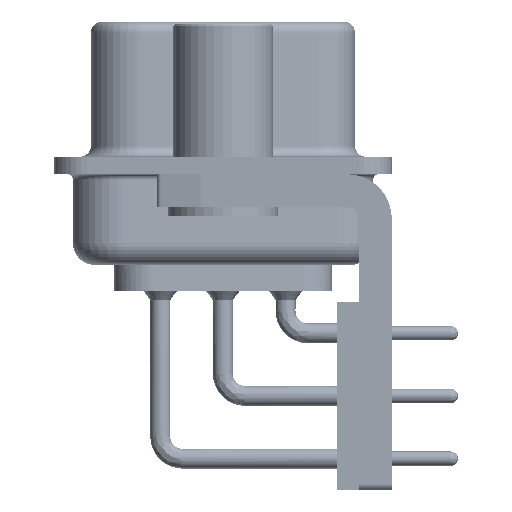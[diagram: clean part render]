
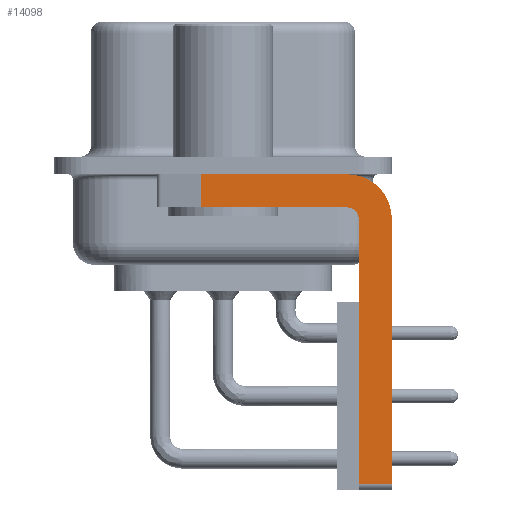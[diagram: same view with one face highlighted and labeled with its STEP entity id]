
A CAD part, left-side view. The second image highlights one B-rep face of the part: STEP entity #14098.
In plain terms, the highlighted planar face has unit normal (-1, 0, 0).
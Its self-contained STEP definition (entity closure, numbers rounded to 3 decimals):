
#279 = ORIENTED_EDGE ( 'NONE', *, *, #39820, .F. ) ;
#511 = EDGE_CURVE ( 'NONE', #20341, #10625, #32950, .T. ) ;
#591 = DIRECTION ( 'NONE',  ( -1., 0., 0. ) ) ;
#1007 = DIRECTION ( 'NONE',  ( 0., 0., -1. ) ) ;
#1360 = VERTEX_POINT ( 'NONE', #37572 ) ;
#3032 = VERTEX_POINT ( 'NONE', #11456 ) ;
#4516 = DIRECTION ( 'NONE',  ( 0., -1., 0. ) ) ;
#6173 = ORIENTED_EDGE ( 'NONE', *, *, #35330, .F. ) ;
#7024 = VECTOR ( 'NONE', #4516, 1000. ) ;
#7232 = DIRECTION ( 'NONE',  ( 0., 0., -1. ) ) ;
#7385 = CARTESIAN_POINT ( 'NONE',  ( -2.9, -5.65, -2.4 ) ) ;
#7639 = CARTESIAN_POINT ( 'NONE',  ( -2.9, -6.15, -2.4 ) ) ;
#7885 = CARTESIAN_POINT ( 'NONE',  ( -2.9, -7.65, -2.4 ) ) ;
#8043 = CARTESIAN_POINT ( 'NONE',  ( -2.9, -5.65, -0.4 ) ) ;
#10420 = AXIS2_PLACEMENT_3D ( 'NONE', #30275, #16977, #40250 ) ;
#10625 = VERTEX_POINT ( 'NONE', #34859 ) ;
#10697 = DIRECTION ( 'NONE',  ( 0., 0., -1. ) ) ;
#10797 = EDGE_CURVE ( 'NONE', #16590, #41067, #23030, .T. ) ;
#11065 = EDGE_CURVE ( 'NONE', #16590, #10625, #13552, .T. ) ;
#11456 = CARTESIAN_POINT ( 'NONE',  ( -2.9, -5.65, -1.9 ) ) ;
#13552 = LINE ( 'NONE', #17328, #39114 ) ;
#13610 = PLANE ( 'NONE',  #10420 ) ;
#13932 = ORIENTED_EDGE ( 'NONE', *, *, #35905, .T. ) ;
#13937 = DIRECTION ( 'NONE',  ( 0., -1., 0. ) ) ;
#14098 = ADVANCED_FACE ( 'NONE', ( #29364 ), #13610, .F. ) ;
#14956 = ORIENTED_EDGE ( 'NONE', *, *, #34582, .F. ) ;
#15943 = VECTOR ( 'NONE', #7232, 1000. ) ;
#16411 = ORIENTED_EDGE ( 'NONE', *, *, #11065, .T. ) ;
#16590 = VERTEX_POINT ( 'NONE', #34690 ) ;
#16977 = DIRECTION ( 'NONE',  ( 1., 0., 0. ) ) ;
#17328 = CARTESIAN_POINT ( 'NONE',  ( -2.9, -5.65, -14.45 ) ) ;
#17830 = VERTEX_POINT ( 'NONE', #24993 ) ;
#18356 = CIRCLE ( 'NONE', #28005, 2. ) ;
#20341 = VERTEX_POINT ( 'NONE', #41490 ) ;
#20487 = AXIS2_PLACEMENT_3D ( 'NONE', #20669, #591, #24038 ) ;
#20669 = CARTESIAN_POINT ( 'NONE',  ( -2.9, -5.65, -2.4 ) ) ;
#21208 = CARTESIAN_POINT ( 'NONE',  ( -2.9, 3., -0.4 ) ) ;
#21268 = ORIENTED_EDGE ( 'NONE', *, *, #40990, .F. ) ;
#21696 = VERTEX_POINT ( 'NONE', #8043 ) ;
#23030 = LINE ( 'NONE', #25973, #41695 ) ;
#23339 = EDGE_LOOP ( 'NONE', ( #6173, #13932, #279, #14956, #37537, #16411, #38162, #21268 ) ) ;
#23441 = VECTOR ( 'NONE', #24476, 1000. ) ;
#24038 = DIRECTION ( 'NONE',  ( 0., 0., 1. ) ) ;
#24105 = VECTOR ( 'NONE', #1007, 1000. ) ;
#24476 = DIRECTION ( 'NONE',  ( 0., 1., 0. ) ) ;
#24993 = CARTESIAN_POINT ( 'NONE',  ( -2.9, 0.978, -1.9 ) ) ;
#25835 = DIRECTION ( 'NONE',  ( 0., 0., 1. ) ) ;
#25973 = CARTESIAN_POINT ( 'NONE',  ( -2.9, -6.15, -14.7 ) ) ;
#28005 = AXIS2_PLACEMENT_3D ( 'NONE', #7385, #30782, #10697 ) ;
#29364 = FACE_OUTER_BOUND ( 'NONE', #23339, .T. ) ;
#30275 = CARTESIAN_POINT ( 'NONE',  ( -2.9, -5.65, -2.4 ) ) ;
#30782 = DIRECTION ( 'NONE',  ( 1., 0., 0. ) ) ;
#31570 = LINE ( 'NONE', #40591, #15943 ) ;
#32289 = LINE ( 'NONE', #37705, #23441 ) ;
#32950 = LINE ( 'NONE', #7885, #24105 ) ;
#34582 = EDGE_CURVE ( 'NONE', #41067, #3032, #35891, .T. ) ;
#34690 = CARTESIAN_POINT ( 'NONE',  ( -2.9, -6.15, -14.45 ) ) ;
#34859 = CARTESIAN_POINT ( 'NONE',  ( -2.9, -7.65, -14.45 ) ) ;
#35330 = EDGE_CURVE ( 'NONE', #1360, #21696, #42475, .T. ) ;
#35891 = CIRCLE ( 'NONE', #20487, 0.5 ) ;
#35905 = EDGE_CURVE ( 'NONE', #1360, #17830, #31570, .T. ) ;
#37537 = ORIENTED_EDGE ( 'NONE', *, *, #10797, .F. ) ;
#37572 = CARTESIAN_POINT ( 'NONE',  ( -2.9, 0.978, -0.4 ) ) ;
#37705 = CARTESIAN_POINT ( 'NONE',  ( -2.9, -5.65, -1.9 ) ) ;
#38162 = ORIENTED_EDGE ( 'NONE', *, *, #511, .F. ) ;
#39114 = VECTOR ( 'NONE', #13937, 1000. ) ;
#39820 = EDGE_CURVE ( 'NONE', #3032, #17830, #32289, .T. ) ;
#40250 = DIRECTION ( 'NONE',  ( 0., 0., -1. ) ) ;
#40591 = CARTESIAN_POINT ( 'NONE',  ( -2.9, 0.978, -1.9 ) ) ;
#40990 = EDGE_CURVE ( 'NONE', #21696, #20341, #18356, .T. ) ;
#41067 = VERTEX_POINT ( 'NONE', #7639 ) ;
#41490 = CARTESIAN_POINT ( 'NONE',  ( -2.9, -7.65, -2.4 ) ) ;
#41695 = VECTOR ( 'NONE', #25835, 1000. ) ;
#42475 = LINE ( 'NONE', #21208, #7024 ) ;
